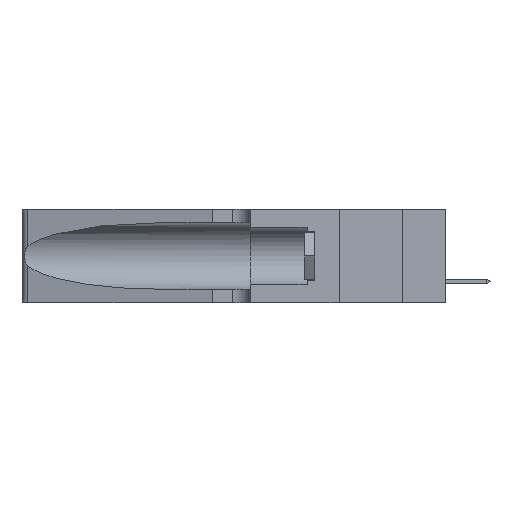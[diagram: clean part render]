
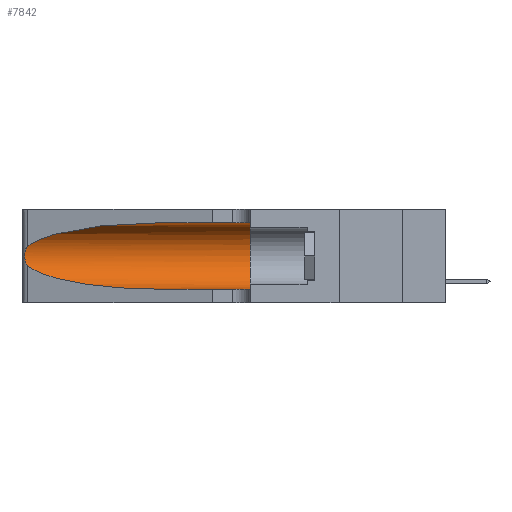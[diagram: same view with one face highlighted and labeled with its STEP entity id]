
A CAD part, left-side view. The second image highlights one B-rep face of the part: STEP entity #7842.
In plain terms, the highlighted cylindrical face has radius 3.308 mm (diameter 6.617 mm), a partial arc.
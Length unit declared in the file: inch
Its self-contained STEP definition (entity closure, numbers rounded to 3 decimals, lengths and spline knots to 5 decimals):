
#84 = CARTESIAN_POINT ( 'NONE',  ( 0.26075, 1.23896, 0.178 ) ) ;
#127 = EDGE_CURVE ( 'NONE', #18967, #19193, #1024, .T. ) ;
#483 = CARTESIAN_POINT ( 'NONE',  ( 0.1305, 0.72297, 0.05475 ) ) ;
#733 = CARTESIAN_POINT ( 'NONE',  ( 0.1305, 0.35, 0.31525 ) ) ;
#792 = AXIS2_PLACEMENT_3D ( 'NONE', #8049, #18427, #6420 ) ;
#1024 = LINE ( 'NONE', #16503, #4706 ) ;
#1595 = CARTESIAN_POINT ( 'NONE',  ( 0.25639, 1.23186, 0.15144 ) ) ;
#1714 = CARTESIAN_POINT ( 'NONE',  ( 0.25789, 1.23486, 0.15765 ) ) ;
#2681 = VERTEX_POINT ( 'NONE', #6783 ) ;
#2699 = CARTESIAN_POINT ( 'NONE',  ( 0.1305, 0.72297, 0.31525 ) ) ;
#3000 = CARTESIAN_POINT ( 'NONE',  ( 0.25487, 1.22718, 0.22369 ) ) ;
#3063 = CARTESIAN_POINT ( 'NONE',  ( 0.25555, 1.22993, 0.14849 ) ) ;
#3159 = DIRECTION ( 'NONE',  ( 0., -1., 0. ) ) ;
#3262 = CARTESIAN_POINT ( 'NONE',  ( 0.25487, 1.22718, 0.14631 ) ) ;
#3853 = CIRCLE ( 'NONE', #10068, 0.13025 ) ;
#4175 = FACE_OUTER_BOUND ( 'NONE', #6928, .T. ) ;
#4229 = ORIENTED_EDGE ( 'NONE', *, *, #127, .T. ) ;
#4275 = VERTEX_POINT ( 'NONE', #14896 ) ;
#4601 = ORIENTED_EDGE ( 'NONE', *, *, #13580, .F. ) ;
#4706 = VECTOR ( 'NONE', #3159, 39.37008 ) ;
#4746 = CARTESIAN_POINT ( 'NONE',  ( 0.25787, 1.23484, 0.2124 ) ) ;
#5272 = DIRECTION ( 'NONE',  ( 0., 1., 0. ) ) ;
#5858 = EDGE_CURVE ( 'NONE', #2681, #4275, #8752, .T. ) ;
#6212 = CARTESIAN_POINT ( 'NONE',  ( 0.25639, 1.23184, 0.21858 ) ) ;
#6420 = DIRECTION ( 'NONE',  ( 0., 0., -1. ) ) ;
#6570 = CARTESIAN_POINT ( 'NONE',  ( 0.1305, 0.72297, 0.31525 ) ) ;
#6611 = CARTESIAN_POINT ( 'NONE',  ( 0.25487, 1.22718, 0.14631 ) ) ;
#6783 = CARTESIAN_POINT ( 'NONE',  ( 0.25487, 1.22718, 0.22369 ) ) ;
#6928 = EDGE_LOOP ( 'NONE', ( #8187, #17552, #8160, #4229, #4601, #6959 ) ) ;
#6959 = ORIENTED_EDGE ( 'NONE', *, *, #14725, .F. ) ;
#7257 = DIRECTION ( 'NONE',  ( 0., -1., 0. ) ) ;
#7842 = ADVANCED_FACE ( 'NONE', ( #4175 ), #14396, .F. ) ;
#8049 = CARTESIAN_POINT ( 'NONE',  ( 0.1305, 1.61858, 0.185 ) ) ;
#8160 = ORIENTED_EDGE ( 'NONE', *, *, #19096, .T. ) ;
#8187 = ORIENTED_EDGE ( 'NONE', *, *, #9030, .T. ) ;
#8390 = CARTESIAN_POINT ( 'NONE',  ( 0.2373, 1.15595, 0.28018 ) ) ;
#8589 = CARTESIAN_POINT ( 'NONE',  ( 0.1305, 1.61858, 0.31525 ) ) ;
#8752 = B_SPLINE_CURVE_WITH_KNOTS ( 'NONE', 3,
 ( #3000, #17822, #6212, #4746, #13372, #8952, #16358, #84, #15067, #9022, #1714, #1595, #3063, #3262 ),
 .UNSPECIFIED., .F., .F.,
 ( 4, 2, 2, 2, 2, 2, 4 ),
 ( 0., 0.00027, 0.00053, 0.00107, 0.0016, 0.00187, 0.00214 ),
 .UNSPECIFIED. ) ;
#8952 = CARTESIAN_POINT ( 'NONE',  ( 0.26018, 1.23835, 0.19895 ) ) ;
#9022 = CARTESIAN_POINT ( 'NONE',  ( 0.25856, 1.23593, 0.16098 ) ) ;
#9030 = EDGE_CURVE ( 'NONE', #10683, #2681, #15778, .T. ) ;
#9803 = DIRECTION ( 'NONE',  ( 0., 0., 1. ) ) ;
#10068 = AXIS2_PLACEMENT_3D ( 'NONE', #14219, #5272, #9803 ) ;
#10280 =( BOUNDED_CURVE ( )  B_SPLINE_CURVE ( 3, ( #6611, #18496, #15466, #11101 ),
 .UNSPECIFIED., .F., .F. ) 
 B_SPLINE_CURVE_WITH_KNOTS ( ( 4, 4 ),
 ( 3.44316, 4.71239 ),
 .UNSPECIFIED. ) 
 CURVE ( )  GEOMETRIC_REPRESENTATION_ITEM ( )  RATIONAL_B_SPLINE_CURVE ( ( 1., 0.87, 0.87, 1. ) ) 
 REPRESENTATION_ITEM ( '' )  );
#10683 = VERTEX_POINT ( 'NONE', #2699 ) ;
#11101 = CARTESIAN_POINT ( 'NONE',  ( 0.1305, 0.72297, 0.05475 ) ) ;
#11906 = LINE ( 'NONE', #8589, #16315 ) ;
#13074 = VERTEX_POINT ( 'NONE', #733 ) ;
#13372 = CARTESIAN_POINT ( 'NONE',  ( 0.25854, 1.2359, 0.20912 ) ) ;
#13580 = EDGE_CURVE ( 'NONE', #13074, #19193, #3853, .T. ) ;
#14219 = CARTESIAN_POINT ( 'NONE',  ( 0.1305, 0.35, 0.185 ) ) ;
#14396 = CYLINDRICAL_SURFACE ( 'NONE', #792, 0.13025 ) ;
#14725 = EDGE_CURVE ( 'NONE', #10683, #13074, #11906, .T. ) ;
#14896 = CARTESIAN_POINT ( 'NONE',  ( 0.25487, 1.22718, 0.14631 ) ) ;
#15067 = CARTESIAN_POINT ( 'NONE',  ( 0.26017, 1.23833, 0.17102 ) ) ;
#15466 = CARTESIAN_POINT ( 'NONE',  ( 0.18966, 0.96281, 0.05475 ) ) ;
#15778 =( BOUNDED_CURVE ( )  B_SPLINE_CURVE ( 3, ( #6570, #16962, #8390, #17461 ),
 .UNSPECIFIED., .F., .T. ) 
 B_SPLINE_CURVE_WITH_KNOTS ( ( 4, 4 ),
 ( 1.5708, 2.84003 ),
 .UNSPECIFIED. ) 
 CURVE ( )  GEOMETRIC_REPRESENTATION_ITEM ( )  RATIONAL_B_SPLINE_CURVE ( ( 1., 0.87, 0.87, 1. ) ) 
 REPRESENTATION_ITEM ( '' )  );
#16315 = VECTOR ( 'NONE', #7257, 39.37008 ) ;
#16358 = CARTESIAN_POINT ( 'NONE',  ( 0.26075, 1.23896, 0.19203 ) ) ;
#16503 = CARTESIAN_POINT ( 'NONE',  ( 0.1305, 1.61858, 0.05475 ) ) ;
#16962 = CARTESIAN_POINT ( 'NONE',  ( 0.18966, 0.96281, 0.31525 ) ) ;
#17252 = CARTESIAN_POINT ( 'NONE',  ( 0.1305, 0.35, 0.05475 ) ) ;
#17461 = CARTESIAN_POINT ( 'NONE',  ( 0.25487, 1.22718, 0.22369 ) ) ;
#17552 = ORIENTED_EDGE ( 'NONE', *, *, #5858, .T. ) ;
#17822 = CARTESIAN_POINT ( 'NONE',  ( 0.25555, 1.22994, 0.2215 ) ) ;
#18427 = DIRECTION ( 'NONE',  ( 0., -1., 0. ) ) ;
#18496 = CARTESIAN_POINT ( 'NONE',  ( 0.2373, 1.15595, 0.08982 ) ) ;
#18967 = VERTEX_POINT ( 'NONE', #483 ) ;
#19096 = EDGE_CURVE ( 'NONE', #4275, #18967, #10280, .T. ) ;
#19193 = VERTEX_POINT ( 'NONE', #17252 ) ;
